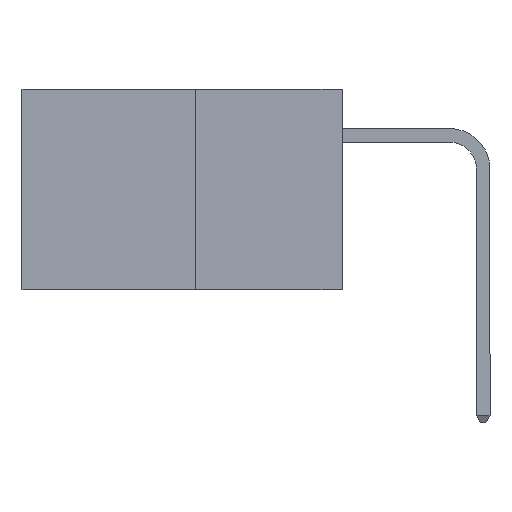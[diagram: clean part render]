
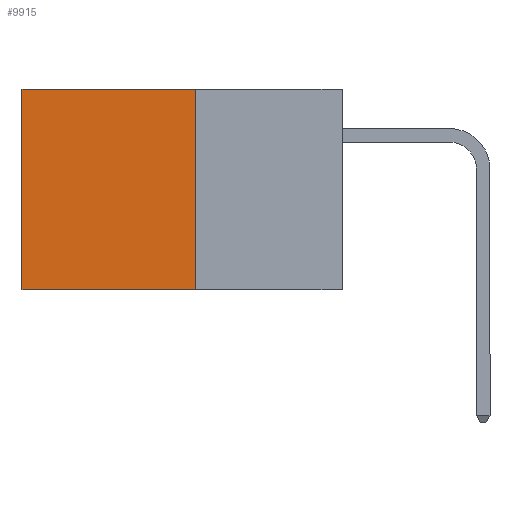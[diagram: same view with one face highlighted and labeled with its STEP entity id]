
A CAD part, left-side view. The second image highlights one B-rep face of the part: STEP entity #9915.
In plain terms, the highlighted planar face has unit normal (-1, 0, 0).
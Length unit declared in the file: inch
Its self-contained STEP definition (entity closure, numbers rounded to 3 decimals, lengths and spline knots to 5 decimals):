
#293 = CARTESIAN_POINT ( 'NONE',  ( 0.277, 0.59, 0. ) ) ;
#942 = DIRECTION ( 'NONE',  ( 0., 0., -1. ) ) ;
#1467 = EDGE_LOOP ( 'NONE', ( #3871, #4443, #4509, #4616 ) ) ;
#1772 = CARTESIAN_POINT ( 'NONE',  ( 0.277, 0.27, -0.37 ) ) ;
#1925 = VERTEX_POINT ( 'NONE', #5144 ) ;
#1984 = LINE ( 'NONE', #8137, #4241 ) ;
#2068 = DIRECTION ( 'NONE',  ( 1., 0., 0. ) ) ;
#2196 = CARTESIAN_POINT ( 'NONE',  ( 0.277, 0.59, -0.37 ) ) ;
#3390 = CARTESIAN_POINT ( 'NONE',  ( 0.277, 0.27, 0. ) ) ;
#3395 = EDGE_CURVE ( 'NONE', #4458, #1925, #10461, .T. ) ;
#3537 = VECTOR ( 'NONE', #8935, 39.37008 ) ;
#3871 = ORIENTED_EDGE ( 'NONE', *, *, #11163, .T. ) ;
#4241 = VECTOR ( 'NONE', #942, 39.37008 ) ;
#4246 = CARTESIAN_POINT ( 'NONE',  ( 0.277, 0.27, -0.37 ) ) ;
#4443 = ORIENTED_EDGE ( 'NONE', *, *, #3395, .F. ) ;
#4458 = VERTEX_POINT ( 'NONE', #4246 ) ;
#4509 = ORIENTED_EDGE ( 'NONE', *, *, #4626, .F. ) ;
#4510 = VERTEX_POINT ( 'NONE', #3390 ) ;
#4616 = ORIENTED_EDGE ( 'NONE', *, *, #7585, .T. ) ;
#4626 = EDGE_CURVE ( 'NONE', #4510, #4458, #1984, .T. ) ;
#4755 = LINE ( 'NONE', #2196, #5039 ) ;
#5039 = VECTOR ( 'NONE', #8463, 39.37008 ) ;
#5144 = CARTESIAN_POINT ( 'NONE',  ( 0.277, 0.59, -0.37 ) ) ;
#5749 = PLANE ( 'NONE',  #9626 ) ;
#7271 = FACE_OUTER_BOUND ( 'NONE', #1467, .T. ) ;
#7317 = LINE ( 'NONE', #9058, #9295 ) ;
#7512 = CARTESIAN_POINT ( 'NONE',  ( 0.277, 0.27, -0.37 ) ) ;
#7585 = EDGE_CURVE ( 'NONE', #4510, #11212, #7317, .T. ) ;
#8137 = CARTESIAN_POINT ( 'NONE',  ( 0.277, 0.27, -0.37 ) ) ;
#8351 = DIRECTION ( 'NONE',  ( 0., 0., -1. ) ) ;
#8463 = DIRECTION ( 'NONE',  ( 0., 0., -1. ) ) ;
#8935 = DIRECTION ( 'NONE',  ( 0., 1., 0. ) ) ;
#9058 = CARTESIAN_POINT ( 'NONE',  ( 0.277, 0.27, 0. ) ) ;
#9067 = DIRECTION ( 'NONE',  ( 0., 1., 0. ) ) ;
#9295 = VECTOR ( 'NONE', #9067, 39.37008 ) ;
#9626 = AXIS2_PLACEMENT_3D ( 'NONE', #7512, #2068, #8351 ) ;
#9915 = ADVANCED_FACE ( 'NONE', ( #7271 ), #5749, .F. ) ;
#10461 = LINE ( 'NONE', #1772, #3537 ) ;
#11163 = EDGE_CURVE ( 'NONE', #11212, #1925, #4755, .T. ) ;
#11212 = VERTEX_POINT ( 'NONE', #293 ) ;
